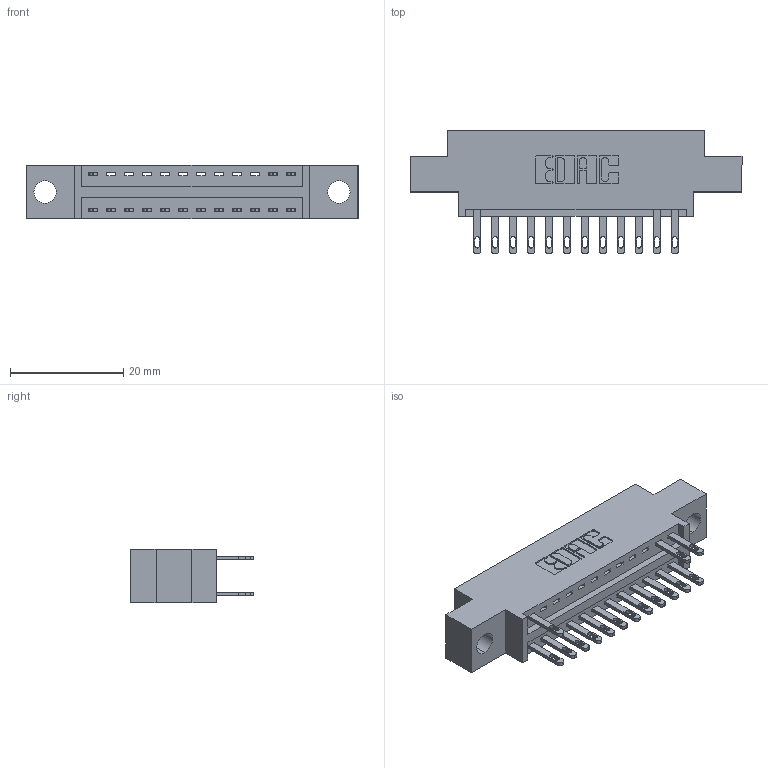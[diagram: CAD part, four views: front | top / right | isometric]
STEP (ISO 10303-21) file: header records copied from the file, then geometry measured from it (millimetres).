
FILE_DESCRIPTION (( 'STEP AP203' ), '1' );
FILE_NAME ('346-024-500-804.STEP', '2018-08-21T02:42:43', ( '' ), ( '' ), 'SwSTEP 2.0', 'SolidWorks 2016', '' );
FILE_SCHEMA (( 'CONFIG_CONTROL_DESIGN' ));
Length unit declared in the file: inch
Products named in the file (3): 346-024-500-804; 346 Part_0.170 Offset - 0.156 Dia-TH; 345-292-001_345-293-100
Assembly tree (16 placements, depth 2):
  346-024-500-804
    346 Part_0.170 Offset - 0.156 Dia-TH
    345-292-001_345-293-100  x15
Bounding box: 58.67 x 21.84 x 9.4 mm (x, y, z)
Volume: 5210.8 mm3; surface area: 6374 mm2
Topology: 16 solids, 16 shells, 900 faces, 2735 edges, 1822 vertices
Faces by surface type: plane 560, cylinder 340
Entity records: 11647 total; most frequent: CARTESIAN_POINT 1999, ORIENTED_EDGE 1942, DIRECTION 1805, EDGE_CURVE 971, LINE 787, VECTOR 787, VERTEX_POINT 646, AXIS2_PLACEMENT_3D 509
